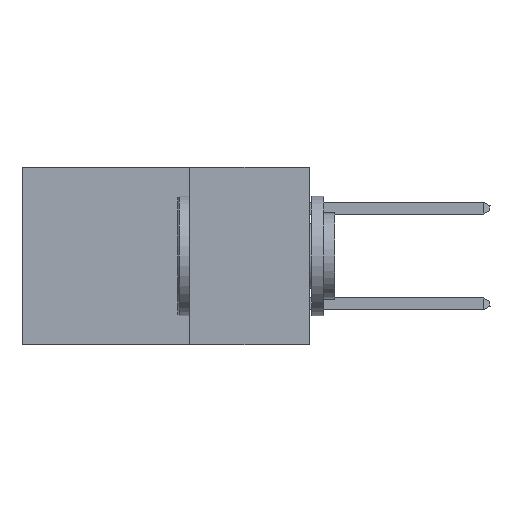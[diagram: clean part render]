
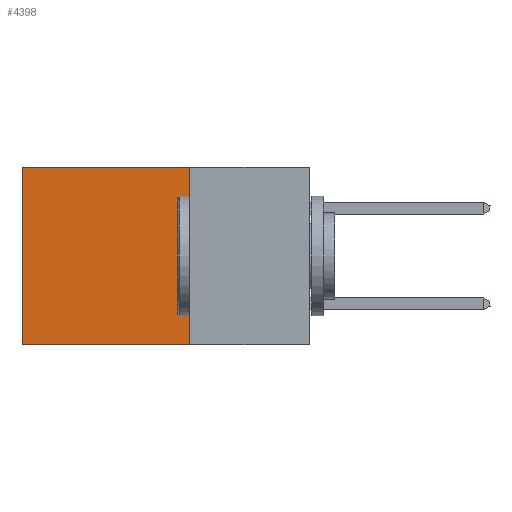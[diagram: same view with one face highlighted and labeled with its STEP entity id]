
A CAD part, left-side view. The second image highlights one B-rep face of the part: STEP entity #4398.
In plain terms, the highlighted planar face has unit normal (-1, 0, 0).
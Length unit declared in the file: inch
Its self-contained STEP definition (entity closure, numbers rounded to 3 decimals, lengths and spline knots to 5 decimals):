
#79 = CARTESIAN_POINT ( 'NONE',  ( 0.2875, 0.25, -0.37 ) ) ;
#741 = VERTEX_POINT ( 'NONE', #6260 ) ;
#1019 = CARTESIAN_POINT ( 'NONE',  ( 0.2875, 0.6, 0. ) ) ;
#1215 = VERTEX_POINT ( 'NONE', #79 ) ;
#1653 = DIRECTION ( 'NONE',  ( 0., 0., -1. ) ) ;
#1666 = DIRECTION ( 'NONE',  ( 1., 0., 0. ) ) ;
#1678 = CARTESIAN_POINT ( 'NONE',  ( 0.2875, 0.25, 0. ) ) ;
#1858 = PLANE ( 'NONE',  #4913 ) ;
#1888 = VECTOR ( 'NONE', #8708, 39.37008 ) ;
#2108 = LINE ( 'NONE', #4490, #9843 ) ;
#2248 = LINE ( 'NONE', #5352, #6598 ) ;
#2409 = LINE ( 'NONE', #3306, #1888 ) ;
#2580 = EDGE_CURVE ( 'NONE', #1215, #741, #2248, .T. ) ;
#3306 = CARTESIAN_POINT ( 'NONE',  ( 0.2875, 0.6, 0. ) ) ;
#3458 = EDGE_CURVE ( 'NONE', #7311, #1215, #4425, .T. ) ;
#3952 = EDGE_CURVE ( 'NONE', #7311, #4503, #2108, .T. ) ;
#4398 = ADVANCED_FACE ( 'NONE', ( #7542 ), #1858, .F. ) ;
#4425 = LINE ( 'NONE', #7186, #8557 ) ;
#4430 = EDGE_LOOP ( 'NONE', ( #7143, #9866, #7030, #9337 ) ) ;
#4490 = CARTESIAN_POINT ( 'NONE',  ( 0.2875, 0.25, 0. ) ) ;
#4501 = DIRECTION ( 'NONE',  ( 0., 1., 0. ) ) ;
#4503 = VERTEX_POINT ( 'NONE', #1019 ) ;
#4913 = AXIS2_PLACEMENT_3D ( 'NONE', #1678, #1666, #1653 ) ;
#5352 = CARTESIAN_POINT ( 'NONE',  ( 0.2875, 0.25, -0.37 ) ) ;
#5520 = DIRECTION ( 'NONE',  ( 0., 1., 0. ) ) ;
#6260 = CARTESIAN_POINT ( 'NONE',  ( 0.2875, 0.6, -0.37 ) ) ;
#6598 = VECTOR ( 'NONE', #5520, 39.37008 ) ;
#7030 = ORIENTED_EDGE ( 'NONE', *, *, #3458, .F. ) ;
#7143 = ORIENTED_EDGE ( 'NONE', *, *, #8713, .T. ) ;
#7146 = DIRECTION ( 'NONE',  ( 0., 0., -1. ) ) ;
#7186 = CARTESIAN_POINT ( 'NONE',  ( 0.2875, 0.25, 0. ) ) ;
#7311 = VERTEX_POINT ( 'NONE', #10051 ) ;
#7542 = FACE_OUTER_BOUND ( 'NONE', #4430, .T. ) ;
#8557 = VECTOR ( 'NONE', #7146, 39.37008 ) ;
#8708 = DIRECTION ( 'NONE',  ( 0., 0., -1. ) ) ;
#8713 = EDGE_CURVE ( 'NONE', #4503, #741, #2409, .T. ) ;
#9337 = ORIENTED_EDGE ( 'NONE', *, *, #3952, .T. ) ;
#9843 = VECTOR ( 'NONE', #4501, 39.37008 ) ;
#9866 = ORIENTED_EDGE ( 'NONE', *, *, #2580, .F. ) ;
#10051 = CARTESIAN_POINT ( 'NONE',  ( 0.2875, 0.25, 0. ) ) ;
